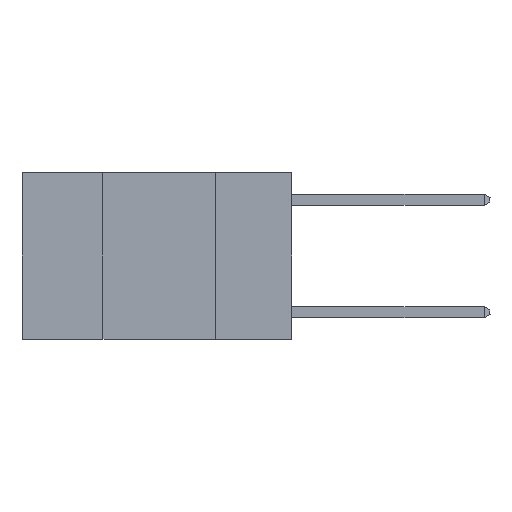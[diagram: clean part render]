
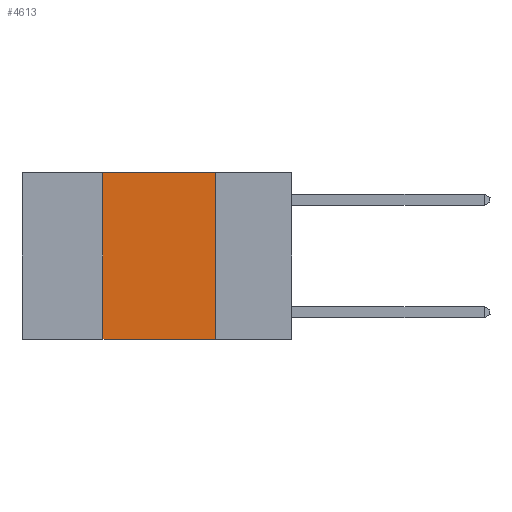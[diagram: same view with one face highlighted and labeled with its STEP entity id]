
A CAD part, left-side view. The second image highlights one B-rep face of the part: STEP entity #4613.
In plain terms, the highlighted planar face has unit normal (-1, 0, 0).
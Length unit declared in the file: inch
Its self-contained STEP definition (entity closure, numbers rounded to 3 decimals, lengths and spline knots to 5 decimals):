
#449 = VERTEX_POINT ( 'NONE', #18776 ) ;
#921 = VECTOR ( 'NONE', #11311, 39.37008 ) ;
#2632 = LINE ( 'NONE', #16640, #14914 ) ;
#2942 = ORIENTED_EDGE ( 'NONE', *, *, #7545, .F. ) ;
#3116 = LINE ( 'NONE', #15505, #13093 ) ;
#3242 = AXIS2_PLACEMENT_3D ( 'NONE', #13212, #11685, #5561 ) ;
#4065 = ORIENTED_EDGE ( 'NONE', *, *, #7114, .T. ) ;
#4613 = ADVANCED_FACE ( 'NONE', ( #16611 ), #8627, .F. ) ;
#5561 = DIRECTION ( 'NONE',  ( 0., 0., -1. ) ) ;
#5919 = ORIENTED_EDGE ( 'NONE', *, *, #13532, .F. ) ;
#5929 = CARTESIAN_POINT ( 'NONE',  ( 0., 0.6, -0.37 ) ) ;
#6907 = CARTESIAN_POINT ( 'NONE',  ( 0., 0.42, 0. ) ) ;
#7114 = EDGE_CURVE ( 'NONE', #10771, #449, #9100, .T. ) ;
#7545 = EDGE_CURVE ( 'NONE', #14062, #19746, #2632, .T. ) ;
#7735 = ORIENTED_EDGE ( 'NONE', *, *, #15050, .F. ) ;
#8033 = DIRECTION ( 'NONE',  ( 0., 0., -1. ) ) ;
#8071 = VECTOR ( 'NONE', #12141, 39.37008 ) ;
#8627 = PLANE ( 'NONE',  #3242 ) ;
#9100 = LINE ( 'NONE', #5929, #8071 ) ;
#10771 = VERTEX_POINT ( 'NONE', #14342 ) ;
#11311 = DIRECTION ( 'NONE',  ( 0., 0., 1. ) ) ;
#11334 = CARTESIAN_POINT ( 'NONE',  ( 0., 0.17, 0. ) ) ;
#11600 = LINE ( 'NONE', #6907, #921 ) ;
#11665 = EDGE_LOOP ( 'NONE', ( #5919, #2942, #7735, #4065 ) ) ;
#11685 = DIRECTION ( 'NONE',  ( 1., 0., 0. ) ) ;
#12141 = DIRECTION ( 'NONE',  ( 0., -1., 0. ) ) ;
#13093 = VECTOR ( 'NONE', #8033, 39.37008 ) ;
#13212 = CARTESIAN_POINT ( 'NONE',  ( 0., 0.6, 0. ) ) ;
#13532 = EDGE_CURVE ( 'NONE', #19746, #449, #3116, .T. ) ;
#14062 = VERTEX_POINT ( 'NONE', #16179 ) ;
#14342 = CARTESIAN_POINT ( 'NONE',  ( 0., 0.42, -0.37 ) ) ;
#14914 = VECTOR ( 'NONE', #20184, 39.37008 ) ;
#15050 = EDGE_CURVE ( 'NONE', #10771, #14062, #11600, .T. ) ;
#15505 = CARTESIAN_POINT ( 'NONE',  ( 0., 0.17, 0. ) ) ;
#16179 = CARTESIAN_POINT ( 'NONE',  ( 0., 0.42, 0. ) ) ;
#16611 = FACE_OUTER_BOUND ( 'NONE', #11665, .T. ) ;
#16640 = CARTESIAN_POINT ( 'NONE',  ( 0., 0.6, 0. ) ) ;
#18776 = CARTESIAN_POINT ( 'NONE',  ( 0., 0.17, -0.37 ) ) ;
#19746 = VERTEX_POINT ( 'NONE', #11334 ) ;
#20184 = DIRECTION ( 'NONE',  ( 0., -1., 0. ) ) ;
